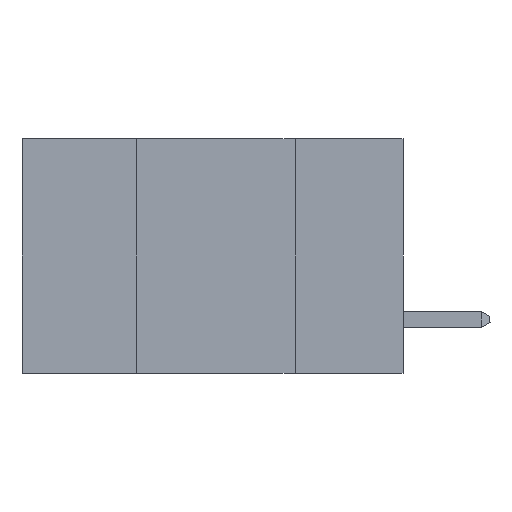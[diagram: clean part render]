
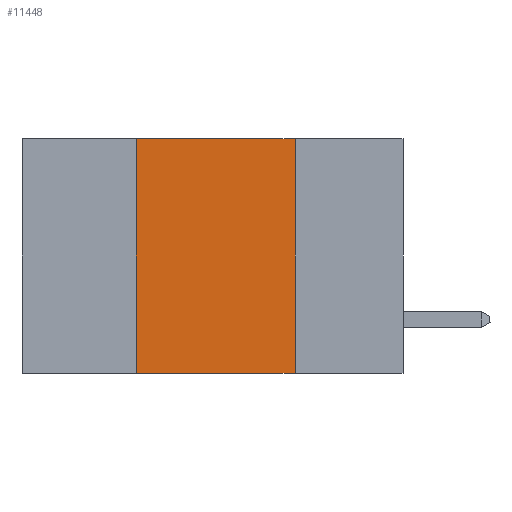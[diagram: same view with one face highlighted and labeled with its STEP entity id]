
A CAD part, left-side view. The second image highlights one B-rep face of the part: STEP entity #11448.
In plain terms, the highlighted planar face has unit normal (-1, 0, 0).
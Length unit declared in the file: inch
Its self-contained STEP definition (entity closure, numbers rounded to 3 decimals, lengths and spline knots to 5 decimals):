
#368 = CARTESIAN_POINT ( 'NONE',  ( 0., 0.42, -0.37 ) ) ;
#790 = FACE_OUTER_BOUND ( 'NONE', #2819, .T. ) ;
#1074 = ORIENTED_EDGE ( 'NONE', *, *, #6754, .F. ) ;
#1123 = DIRECTION ( 'NONE',  ( 0., 0., -1. ) ) ;
#1802 = LINE ( 'NONE', #6773, #5298 ) ;
#2499 = VERTEX_POINT ( 'NONE', #368 ) ;
#2819 = EDGE_LOOP ( 'NONE', ( #1074, #9298, #9172, #8481 ) ) ;
#2960 = DIRECTION ( 'NONE',  ( 0., -1., 0. ) ) ;
#3237 = DIRECTION ( 'NONE',  ( 1., 0., 0. ) ) ;
#3336 = VERTEX_POINT ( 'NONE', #5683 ) ;
#3743 = DIRECTION ( 'NONE',  ( 0., 0., 1. ) ) ;
#3817 = VECTOR ( 'NONE', #9597, 39.37008 ) ;
#3904 = CARTESIAN_POINT ( 'NONE',  ( 0., 0.17, 0. ) ) ;
#5068 = EDGE_CURVE ( 'NONE', #2499, #3336, #10839, .T. ) ;
#5298 = VECTOR ( 'NONE', #2960, 39.37008 ) ;
#5683 = CARTESIAN_POINT ( 'NONE',  ( 0., 0.17, -0.37 ) ) ;
#5753 = CARTESIAN_POINT ( 'NONE',  ( 0., 0.6, -0.37 ) ) ;
#6075 = LINE ( 'NONE', #7344, #8789 ) ;
#6086 = PLANE ( 'NONE',  #10246 ) ;
#6131 = CARTESIAN_POINT ( 'NONE',  ( 0., 0.6, 0. ) ) ;
#6754 = EDGE_CURVE ( 'NONE', #11950, #3336, #6075, .T. ) ;
#6773 = CARTESIAN_POINT ( 'NONE',  ( 0., 0.6, 0. ) ) ;
#7229 = EDGE_CURVE ( 'NONE', #7810, #11950, #1802, .T. ) ;
#7341 = CARTESIAN_POINT ( 'NONE',  ( 0., 0.42, 0. ) ) ;
#7344 = CARTESIAN_POINT ( 'NONE',  ( 0., 0.17, 0. ) ) ;
#7810 = VERTEX_POINT ( 'NONE', #7341 ) ;
#8481 = ORIENTED_EDGE ( 'NONE', *, *, #5068, .T. ) ;
#8789 = VECTOR ( 'NONE', #10343, 39.37008 ) ;
#9172 = ORIENTED_EDGE ( 'NONE', *, *, #11189, .F. ) ;
#9237 = CARTESIAN_POINT ( 'NONE',  ( 0., 0.42, 0. ) ) ;
#9298 = ORIENTED_EDGE ( 'NONE', *, *, #7229, .F. ) ;
#9597 = DIRECTION ( 'NONE',  ( 0., -1., 0. ) ) ;
#10246 = AXIS2_PLACEMENT_3D ( 'NONE', #6131, #3237, #1123 ) ;
#10343 = DIRECTION ( 'NONE',  ( 0., 0., -1. ) ) ;
#10686 = LINE ( 'NONE', #9237, #11138 ) ;
#10839 = LINE ( 'NONE', #5753, #3817 ) ;
#11138 = VECTOR ( 'NONE', #3743, 39.37008 ) ;
#11189 = EDGE_CURVE ( 'NONE', #2499, #7810, #10686, .T. ) ;
#11448 = ADVANCED_FACE ( 'NONE', ( #790 ), #6086, .F. ) ;
#11950 = VERTEX_POINT ( 'NONE', #3904 ) ;
